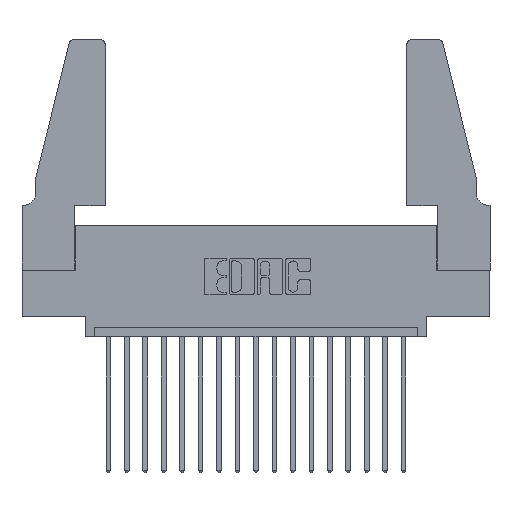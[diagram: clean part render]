
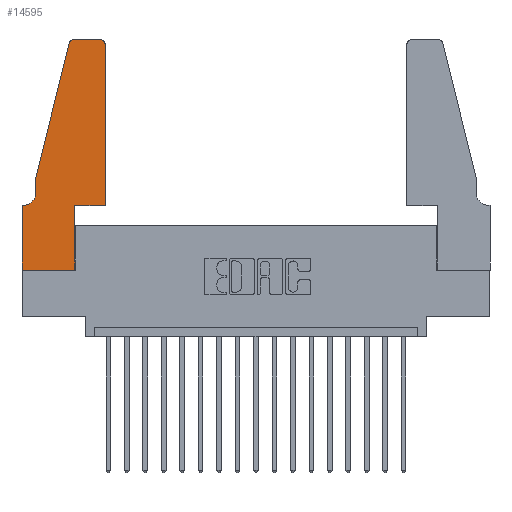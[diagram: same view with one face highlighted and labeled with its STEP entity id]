
A CAD part, top view. The second image highlights one B-rep face of the part: STEP entity #14595.
In plain terms, the highlighted planar face has unit normal (0, 0, 1).
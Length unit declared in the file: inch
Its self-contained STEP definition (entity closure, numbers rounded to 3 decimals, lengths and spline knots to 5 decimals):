
#220 = ORIENTED_EDGE ( 'NONE', *, *, #7625, .T. ) ;
#413 = VECTOR ( 'NONE', #11344, 39.37008 ) ;
#436 = DIRECTION ( 'NONE',  ( -0.239, -0.971, 0. ) ) ;
#553 = LINE ( 'NONE', #1991, #9698 ) ;
#609 = DIRECTION ( 'NONE',  ( 1., 0., 0. ) ) ;
#845 = DIRECTION ( 'NONE',  ( 0., 0., 1. ) ) ;
#859 = AXIS2_PLACEMENT_3D ( 'NONE', #13570, #12232, #9202 ) ;
#918 = AXIS2_PLACEMENT_3D ( 'NONE', #3471, #7505, #609 ) ;
#940 = CARTESIAN_POINT ( 'NONE',  ( 0.2865, 0.35, 0.37 ) ) ;
#1231 = AXIS2_PLACEMENT_3D ( 'NONE', #12211, #845, #13736 ) ;
#1261 = CARTESIAN_POINT ( 'NONE',  ( 0., 0., 0.37 ) ) ;
#1679 = LINE ( 'NONE', #7626, #5921 ) ;
#1707 = CARTESIAN_POINT ( 'NONE',  ( 0., 0.35, 0.37 ) ) ;
#1920 = CARTESIAN_POINT ( 'NONE',  ( 0.284, 1.25, 0.37 ) ) ;
#1991 = CARTESIAN_POINT ( 'NONE',  ( 0., 0., 0.37 ) ) ;
#2144 = ORIENTED_EDGE ( 'NONE', *, *, #7400, .T. ) ;
#2744 = ORIENTED_EDGE ( 'NONE', *, *, #14195, .T. ) ;
#3041 = CIRCLE ( 'NONE', #1231, 0.03 ) ;
#3471 = CARTESIAN_POINT ( 'NONE',  ( 0.4205, 1.22, 0.37 ) ) ;
#3705 = EDGE_CURVE ( 'NONE', #9738, #5883, #12029, .T. ) ;
#3930 = VERTEX_POINT ( 'NONE', #17310 ) ;
#4485 = CARTESIAN_POINT ( 'NONE',  ( 0.0755, 0.5, 0.37 ) ) ;
#4586 = DIRECTION ( 'NONE',  ( -1., 0., 0. ) ) ;
#4664 = EDGE_CURVE ( 'NONE', #17160, #13130, #3041, .T. ) ;
#4808 = CARTESIAN_POINT ( 'NONE',  ( 0.4505, 0.35, 0.37 ) ) ;
#5031 = CIRCLE ( 'NONE', #859, 0.07 ) ;
#5049 = CARTESIAN_POINT ( 'NONE',  ( 0., 0., 0.37 ) ) ;
#5789 = CARTESIAN_POINT ( 'NONE',  ( 0.0755, 0.5, 0.37 ) ) ;
#5883 = VERTEX_POINT ( 'NONE', #10675 ) ;
#5921 = VECTOR ( 'NONE', #9068, 39.37008 ) ;
#6377 = VERTEX_POINT ( 'NONE', #17888 ) ;
#6438 = VECTOR ( 'NONE', #12373, 39.37008 ) ;
#6830 = EDGE_CURVE ( 'NONE', #9970, #3930, #12528, .T. ) ;
#6833 = CARTESIAN_POINT ( 'NONE',  ( 0.4505, 0.35, 0.37 ) ) ;
#7138 = LINE ( 'NONE', #17506, #18060 ) ;
#7139 = ORIENTED_EDGE ( 'NONE', *, *, #15539, .T. ) ;
#7225 = VERTEX_POINT ( 'NONE', #15538 ) ;
#7400 = EDGE_CURVE ( 'NONE', #10824, #7225, #16277, .T. ) ;
#7426 = ORIENTED_EDGE ( 'NONE', *, *, #12923, .T. ) ;
#7505 = DIRECTION ( 'NONE',  ( 0., 0., 1. ) ) ;
#7554 = VECTOR ( 'NONE', #4586, 39.37008 ) ;
#7625 = EDGE_CURVE ( 'NONE', #6377, #10435, #10685, .T. ) ;
#7626 = CARTESIAN_POINT ( 'NONE',  ( 0.2605, 1.25, 0.37 ) ) ;
#7635 = CARTESIAN_POINT ( 'NONE',  ( 0.4505, 1.22, 0.37 ) ) ;
#8037 = DIRECTION ( 'NONE',  ( 0., 0., 1. ) ) ;
#8185 = ORIENTED_EDGE ( 'NONE', *, *, #13641, .T. ) ;
#8775 = CARTESIAN_POINT ( 'NONE',  ( 0.0755, 0.35, 0.37 ) ) ;
#8790 = CARTESIAN_POINT ( 'NONE',  ( 0.0755, 0.42, 0.37 ) ) ;
#9068 = DIRECTION ( 'NONE',  ( -1., 0., 0. ) ) ;
#9151 = EDGE_CURVE ( 'NONE', #10435, #9970, #10396, .T. ) ;
#9202 = DIRECTION ( 'NONE',  ( -1., 0., 0. ) ) ;
#9279 = VECTOR ( 'NONE', #10300, 39.37008 ) ;
#9401 = LINE ( 'NONE', #940, #17439 ) ;
#9425 = EDGE_CURVE ( 'NONE', #3930, #17160, #1679, .T. ) ;
#9471 = DIRECTION ( 'NONE',  ( 1., 0., 0. ) ) ;
#9688 = AXIS2_PLACEMENT_3D ( 'NONE', #1707, #8037, #9471 ) ;
#9698 = VECTOR ( 'NONE', #17692, 39.37008 ) ;
#9738 = VERTEX_POINT ( 'NONE', #1261 ) ;
#9970 = VERTEX_POINT ( 'NONE', #7635 ) ;
#10048 = EDGE_LOOP ( 'NONE', ( #15504, #15005, #11329, #7426, #8185, #2144, #2744, #16747, #7139, #220, #10790, #16165 ) ) ;
#10273 = DIRECTION ( 'NONE',  ( 0., -1., 0. ) ) ;
#10300 = DIRECTION ( 'NONE',  ( 0., 1., 0. ) ) ;
#10396 = LINE ( 'NONE', #4808, #9279 ) ;
#10435 = VERTEX_POINT ( 'NONE', #12841 ) ;
#10675 = CARTESIAN_POINT ( 'NONE',  ( 0.2865, 0., 0.37 ) ) ;
#10685 = LINE ( 'NONE', #6833, #413 ) ;
#10689 = CARTESIAN_POINT ( 'NONE',  ( 0.0055, 0.35, 0.37 ) ) ;
#10790 = ORIENTED_EDGE ( 'NONE', *, *, #9151, .T. ) ;
#10824 = VERTEX_POINT ( 'NONE', #10689 ) ;
#10873 = LINE ( 'NONE', #5789, #13818 ) ;
#11267 = VERTEX_POINT ( 'NONE', #8790 ) ;
#11329 = ORIENTED_EDGE ( 'NONE', *, *, #17134, .T. ) ;
#11344 = DIRECTION ( 'NONE',  ( 1., 0., 0. ) ) ;
#12029 = LINE ( 'NONE', #5049, #6438 ) ;
#12211 = CARTESIAN_POINT ( 'NONE',  ( 0.284, 1.22, 0.37 ) ) ;
#12232 = DIRECTION ( 'NONE',  ( 0., 0., -1. ) ) ;
#12373 = DIRECTION ( 'NONE',  ( 1., 0., 0. ) ) ;
#12528 = CIRCLE ( 'NONE', #918, 0.03 ) ;
#12841 = CARTESIAN_POINT ( 'NONE',  ( 0.4505, 0.35, 0.37 ) ) ;
#12923 = EDGE_CURVE ( 'NONE', #14123, #11267, #10873, .T. ) ;
#13130 = VERTEX_POINT ( 'NONE', #14016 ) ;
#13570 = CARTESIAN_POINT ( 'NONE',  ( 0.0055, 0.42, 0.37 ) ) ;
#13641 = EDGE_CURVE ( 'NONE', #11267, #10824, #5031, .T. ) ;
#13736 = DIRECTION ( 'NONE',  ( 1., 0., 0. ) ) ;
#13818 = VECTOR ( 'NONE', #10273, 39.37008 ) ;
#13820 = DIRECTION ( 'NONE',  ( 0., 1., 0. ) ) ;
#14016 = CARTESIAN_POINT ( 'NONE',  ( 0.25487, 1.22718, 0.37 ) ) ;
#14123 = VERTEX_POINT ( 'NONE', #4485 ) ;
#14195 = EDGE_CURVE ( 'NONE', #7225, #9738, #553, .T. ) ;
#14595 = ADVANCED_FACE ( 'NONE', ( #16390 ), #15324, .T. ) ;
#15005 = ORIENTED_EDGE ( 'NONE', *, *, #4664, .T. ) ;
#15324 = PLANE ( 'NONE',  #9688 ) ;
#15504 = ORIENTED_EDGE ( 'NONE', *, *, #9425, .T. ) ;
#15538 = CARTESIAN_POINT ( 'NONE',  ( 0., 0.35, 0.37 ) ) ;
#15539 = EDGE_CURVE ( 'NONE', #5883, #6377, #9401, .T. ) ;
#16165 = ORIENTED_EDGE ( 'NONE', *, *, #6830, .T. ) ;
#16277 = LINE ( 'NONE', #8775, #7554 ) ;
#16390 = FACE_OUTER_BOUND ( 'NONE', #10048, .T. ) ;
#16747 = ORIENTED_EDGE ( 'NONE', *, *, #3705, .T. ) ;
#17134 = EDGE_CURVE ( 'NONE', #13130, #14123, #7138, .T. ) ;
#17160 = VERTEX_POINT ( 'NONE', #1920 ) ;
#17310 = CARTESIAN_POINT ( 'NONE',  ( 0.4205, 1.25, 0.37 ) ) ;
#17439 = VECTOR ( 'NONE', #13820, 39.37008 ) ;
#17506 = CARTESIAN_POINT ( 'NONE',  ( 0.0755, 0.5, 0.37 ) ) ;
#17692 = DIRECTION ( 'NONE',  ( 0., -1., 0. ) ) ;
#17888 = CARTESIAN_POINT ( 'NONE',  ( 0.2865, 0.35, 0.37 ) ) ;
#18060 = VECTOR ( 'NONE', #436, 39.37008 ) ;
